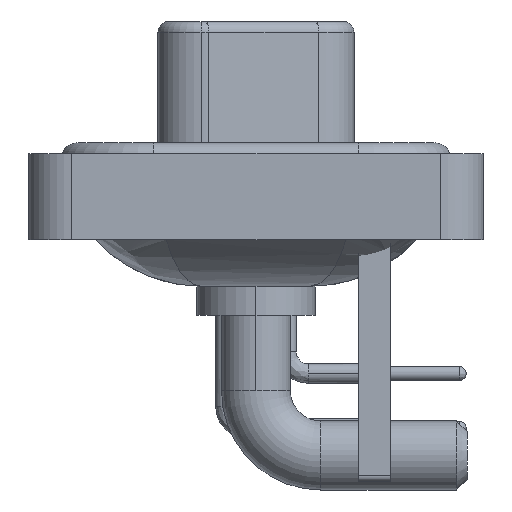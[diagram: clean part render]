
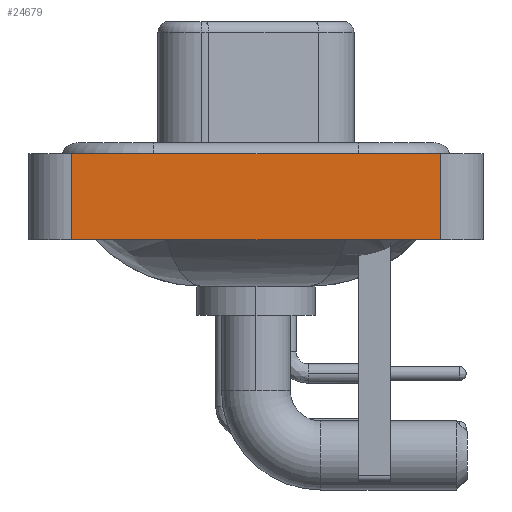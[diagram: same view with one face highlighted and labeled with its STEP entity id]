
A CAD part, left-side view. The second image highlights one B-rep face of the part: STEP entity #24679.
In plain terms, the highlighted planar face has unit normal (-1, 0, 0).
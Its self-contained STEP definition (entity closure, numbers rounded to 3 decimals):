
#31 = DIRECTION ( 'NONE',  ( 0., 0., 1. ) ) ;
#358 = ORIENTED_EDGE ( 'NONE', *, *, #7502, .T. ) ;
#687 = DIRECTION ( 'NONE',  ( -1., 0., 0. ) ) ;
#997 = DIRECTION ( 'NONE',  ( 0., -1., 0. ) ) ;
#1242 = DIRECTION ( 'NONE',  ( 0., -1., 0. ) ) ;
#2008 = LINE ( 'NONE', #21613, #4985 ) ;
#2404 = CARTESIAN_POINT ( 'NONE',  ( -7.35, -8.55, 0.4 ) ) ;
#3389 = LINE ( 'NONE', #7922, #15352 ) ;
#4092 = CARTESIAN_POINT ( 'NONE',  ( -7.35, 8.55, -3.6 ) ) ;
#4339 = AXIS2_PLACEMENT_3D ( 'NONE', #13878, #687, #18421 ) ;
#4789 = CARTESIAN_POINT ( 'NONE',  ( -7.35, 8.55, 0.4 ) ) ;
#4985 = VECTOR ( 'NONE', #31, 1000. ) ;
#5943 = EDGE_CURVE ( 'NONE', #15695, #10397, #3389, .T. ) ;
#7502 = EDGE_CURVE ( 'NONE', #10397, #15389, #2008, .T. ) ;
#7768 = CARTESIAN_POINT ( 'NONE',  ( -7.35, 8.55, -3.6 ) ) ;
#7922 = CARTESIAN_POINT ( 'NONE',  ( -7.35, -8.55, -3.6 ) ) ;
#9062 = LINE ( 'NONE', #4092, #16124 ) ;
#10211 = ORIENTED_EDGE ( 'NONE', *, *, #23209, .F. ) ;
#10397 = VERTEX_POINT ( 'NONE', #26423 ) ;
#11758 = FACE_OUTER_BOUND ( 'NONE', #21903, .T. ) ;
#11981 = ORIENTED_EDGE ( 'NONE', *, *, #5943, .T. ) ;
#12769 = DIRECTION ( 'NONE',  ( 0., 0., 1. ) ) ;
#13878 = CARTESIAN_POINT ( 'NONE',  ( -7.35, -8.55, -3.6 ) ) ;
#15352 = VECTOR ( 'NONE', #997, 1000. ) ;
#15389 = VERTEX_POINT ( 'NONE', #2404 ) ;
#15695 = VERTEX_POINT ( 'NONE', #7768 ) ;
#16124 = VECTOR ( 'NONE', #12769, 1000. ) ;
#18421 = DIRECTION ( 'NONE',  ( 0., 0., 1. ) ) ;
#18844 = LINE ( 'NONE', #23235, #24724 ) ;
#21613 = CARTESIAN_POINT ( 'NONE',  ( -7.35, -8.55, -3.6 ) ) ;
#21903 = EDGE_LOOP ( 'NONE', ( #358, #27312, #10211, #11981 ) ) ;
#22692 = PLANE ( 'NONE',  #4339 ) ;
#23209 = EDGE_CURVE ( 'NONE', #15695, #24586, #9062, .T. ) ;
#23235 = CARTESIAN_POINT ( 'NONE',  ( -7.35, -8.55, 0.4 ) ) ;
#24586 = VERTEX_POINT ( 'NONE', #4789 ) ;
#24679 = ADVANCED_FACE ( 'NONE', ( #11758 ), #22692, .T. ) ;
#24724 = VECTOR ( 'NONE', #1242, 1000. ) ;
#24838 = EDGE_CURVE ( 'NONE', #24586, #15389, #18844, .T. ) ;
#26423 = CARTESIAN_POINT ( 'NONE',  ( -7.35, -8.55, -3.6 ) ) ;
#27312 = ORIENTED_EDGE ( 'NONE', *, *, #24838, .F. ) ;
